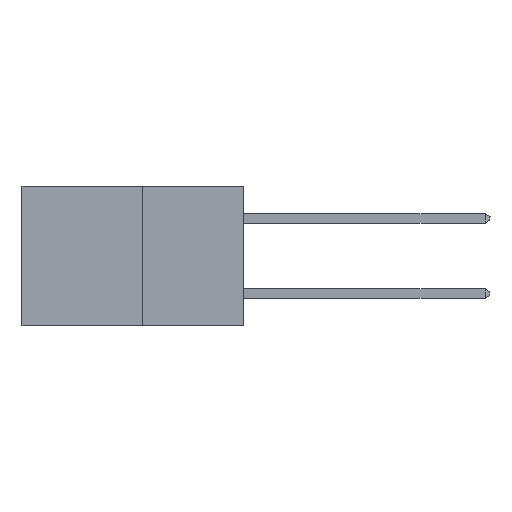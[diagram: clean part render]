
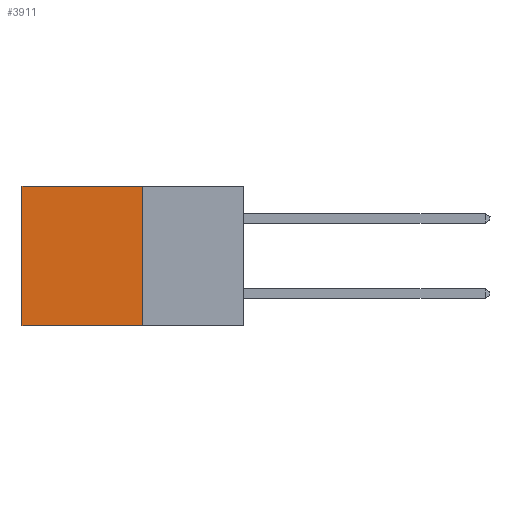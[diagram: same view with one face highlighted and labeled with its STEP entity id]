
A CAD part, left-side view. The second image highlights one B-rep face of the part: STEP entity #3911.
In plain terms, the highlighted planar face has unit normal (-1, 0, 0).
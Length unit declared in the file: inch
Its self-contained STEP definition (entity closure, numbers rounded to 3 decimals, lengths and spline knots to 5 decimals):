
#10 = VECTOR ( 'NONE', #2968, 39.37008 ) ;
#64 = CARTESIAN_POINT ( 'NONE',  ( 0.277, 0.27, -0.37 ) ) ;
#90 = CARTESIAN_POINT ( 'NONE',  ( 0.277, 0.59, -0.37 ) ) ;
#165 = ORIENTED_EDGE ( 'NONE', *, *, #4530, .T. ) ;
#978 = ORIENTED_EDGE ( 'NONE', *, *, #2448, .F. ) ;
#1055 = VERTEX_POINT ( 'NONE', #9545 ) ;
#1312 = LINE ( 'NONE', #13106, #13372 ) ;
#1327 = LINE ( 'NONE', #19419, #13381 ) ;
#2448 = EDGE_CURVE ( 'NONE', #1055, #19023, #1327, .T. ) ;
#2968 = DIRECTION ( 'NONE',  ( 0., 0., -1. ) ) ;
#3165 = CARTESIAN_POINT ( 'NONE',  ( 0.277, 0.59, -0.37 ) ) ;
#3911 = ADVANCED_FACE ( 'NONE', ( #14548 ), #12841, .F. ) ;
#4530 = EDGE_CURVE ( 'NONE', #10072, #18592, #17483, .T. ) ;
#6502 = ORIENTED_EDGE ( 'NONE', *, *, #12685, .T. ) ;
#7345 = EDGE_LOOP ( 'NONE', ( #165, #17126, #978, #6502 ) ) ;
#8222 = DIRECTION ( 'NONE',  ( 0., 0., -1. ) ) ;
#8456 = CARTESIAN_POINT ( 'NONE',  ( 0.277, 0.59, 0. ) ) ;
#9545 = CARTESIAN_POINT ( 'NONE',  ( 0.277, 0.27, 0. ) ) ;
#10072 = VERTEX_POINT ( 'NONE', #8456 ) ;
#10287 = CARTESIAN_POINT ( 'NONE',  ( 0.277, 0.27, -0.37 ) ) ;
#10354 = DIRECTION ( 'NONE',  ( 0., 1., 0. ) ) ;
#10695 = AXIS2_PLACEMENT_3D ( 'NONE', #12981, #12816, #12776 ) ;
#12685 = EDGE_CURVE ( 'NONE', #1055, #10072, #1312, .T. ) ;
#12776 = DIRECTION ( 'NONE',  ( 0., 0., -1. ) ) ;
#12816 = DIRECTION ( 'NONE',  ( 1., 0., 0. ) ) ;
#12841 = PLANE ( 'NONE',  #10695 ) ;
#12981 = CARTESIAN_POINT ( 'NONE',  ( 0.277, 0.27, -0.37 ) ) ;
#13106 = CARTESIAN_POINT ( 'NONE',  ( 0.277, 0.27, 0. ) ) ;
#13372 = VECTOR ( 'NONE', #16108, 39.37008 ) ;
#13381 = VECTOR ( 'NONE', #8222, 39.37008 ) ;
#14548 = FACE_OUTER_BOUND ( 'NONE', #7345, .T. ) ;
#16108 = DIRECTION ( 'NONE',  ( 0., 1., 0. ) ) ;
#17126 = ORIENTED_EDGE ( 'NONE', *, *, #18238, .F. ) ;
#17483 = LINE ( 'NONE', #3165, #10 ) ;
#18238 = EDGE_CURVE ( 'NONE', #19023, #18592, #18929, .T. ) ;
#18471 = VECTOR ( 'NONE', #10354, 39.37008 ) ;
#18592 = VERTEX_POINT ( 'NONE', #90 ) ;
#18929 = LINE ( 'NONE', #10287, #18471 ) ;
#19023 = VERTEX_POINT ( 'NONE', #64 ) ;
#19419 = CARTESIAN_POINT ( 'NONE',  ( 0.277, 0.27, -0.37 ) ) ;
